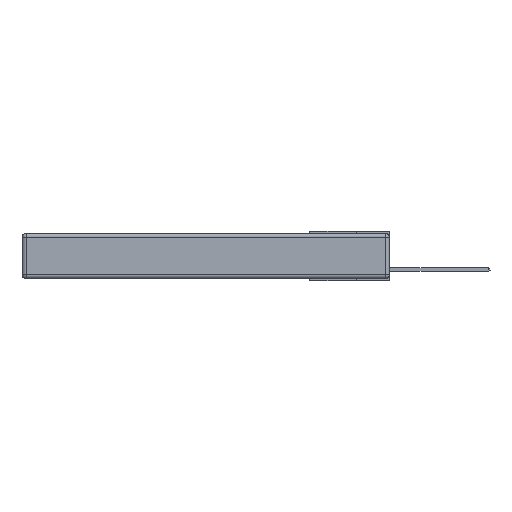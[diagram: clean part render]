
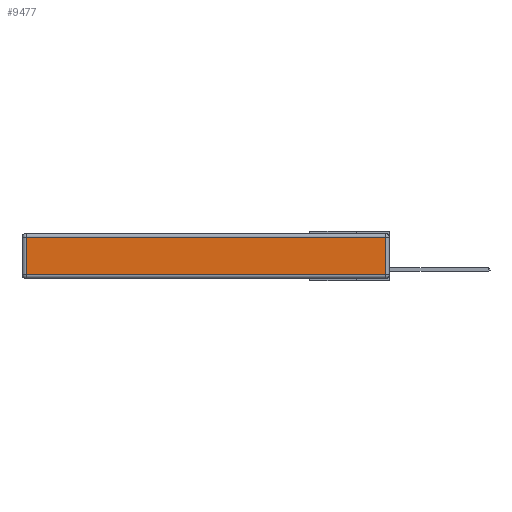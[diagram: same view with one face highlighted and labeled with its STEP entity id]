
A CAD part, left-side view. The second image highlights one B-rep face of the part: STEP entity #9477.
In plain terms, the highlighted planar face has unit normal (-1, 0, 0).
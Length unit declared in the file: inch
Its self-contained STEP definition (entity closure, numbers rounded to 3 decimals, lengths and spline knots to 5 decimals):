
#1613 = EDGE_CURVE ( 'NONE', #11371, #24419, #21622, .T. ) ;
#2115 = CARTESIAN_POINT ( 'NONE',  ( 0., 2.72, -0.313 ) ) ;
#3633 = EDGE_CURVE ( 'NONE', #24419, #21993, #8117, .T. ) ;
#4527 = ORIENTED_EDGE ( 'NONE', *, *, #1613, .T. ) ;
#4746 = CARTESIAN_POINT ( 'NONE',  ( 0., 0.03, -0.313 ) ) ;
#5947 = VECTOR ( 'NONE', #26518, 39.37008 ) ;
#6566 = DIRECTION ( 'NONE',  ( 0., 0., -1. ) ) ;
#7423 = EDGE_LOOP ( 'NONE', ( #4527, #18313, #25754, #16359 ) ) ;
#8117 = LINE ( 'NONE', #13370, #20104 ) ;
#9477 = ADVANCED_FACE ( 'NONE', ( #11379 ), #23729, .T. ) ;
#10807 = DIRECTION ( 'NONE',  ( 0., 0., 1. ) ) ;
#11371 = VERTEX_POINT ( 'NONE', #2115 ) ;
#11379 = FACE_OUTER_BOUND ( 'NONE', #7423, .T. ) ;
#12610 = CARTESIAN_POINT ( 'NONE',  ( 0., 2.72, -0.03 ) ) ;
#13236 = EDGE_CURVE ( 'NONE', #29112, #11371, #22499, .T. ) ;
#13370 = CARTESIAN_POINT ( 'NONE',  ( 0., 0.03, -0.343 ) ) ;
#13666 = EDGE_CURVE ( 'NONE', #21993, #29112, #19111, .T. ) ;
#15328 = CARTESIAN_POINT ( 'NONE',  ( 0., 0.03, -0.03 ) ) ;
#15562 = DIRECTION ( 'NONE',  ( 0., 0., 1. ) ) ;
#15865 = AXIS2_PLACEMENT_3D ( 'NONE', #24040, #26430, #10807 ) ;
#16359 = ORIENTED_EDGE ( 'NONE', *, *, #13236, .T. ) ;
#18313 = ORIENTED_EDGE ( 'NONE', *, *, #3633, .T. ) ;
#19111 = LINE ( 'NONE', #24781, #25453 ) ;
#20104 = VECTOR ( 'NONE', #15562, 39.37008 ) ;
#21622 = LINE ( 'NONE', #30737, #5947 ) ;
#21993 = VERTEX_POINT ( 'NONE', #15328 ) ;
#22499 = LINE ( 'NONE', #25573, #24352 ) ;
#23729 = PLANE ( 'NONE',  #15865 ) ;
#24040 = CARTESIAN_POINT ( 'NONE',  ( 0., 0., -0.343 ) ) ;
#24352 = VECTOR ( 'NONE', #6566, 39.37008 ) ;
#24419 = VERTEX_POINT ( 'NONE', #4746 ) ;
#24554 = DIRECTION ( 'NONE',  ( 0., 1., 0. ) ) ;
#24781 = CARTESIAN_POINT ( 'NONE',  ( 0., 2.75, -0.03 ) ) ;
#25453 = VECTOR ( 'NONE', #24554, 39.37008 ) ;
#25573 = CARTESIAN_POINT ( 'NONE',  ( 0., 2.72, -0.343 ) ) ;
#25754 = ORIENTED_EDGE ( 'NONE', *, *, #13666, .T. ) ;
#26430 = DIRECTION ( 'NONE',  ( -1., 0., 0. ) ) ;
#26518 = DIRECTION ( 'NONE',  ( 0., -1., 0. ) ) ;
#29112 = VERTEX_POINT ( 'NONE', #12610 ) ;
#30737 = CARTESIAN_POINT ( 'NONE',  ( 0., 0., -0.313 ) ) ;
